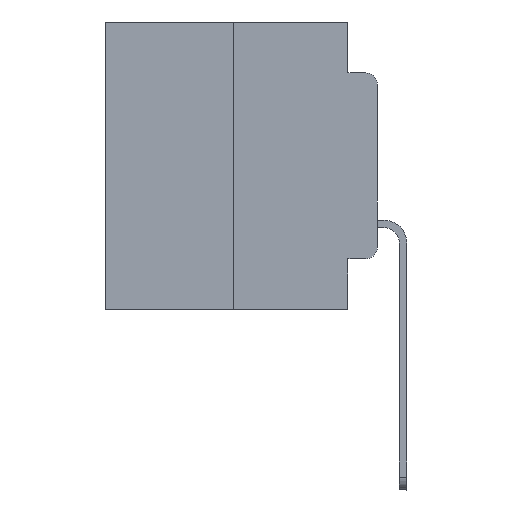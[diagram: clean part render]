
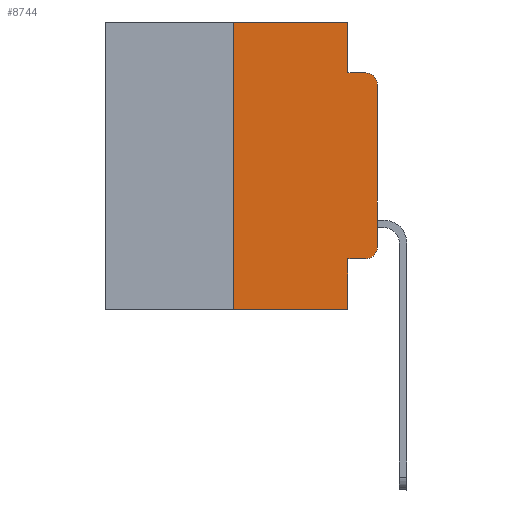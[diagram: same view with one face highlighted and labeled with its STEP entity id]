
A CAD part, left-side view. The second image highlights one B-rep face of the part: STEP entity #8744.
In plain terms, the highlighted planar face has unit normal (-1, 0, 0).
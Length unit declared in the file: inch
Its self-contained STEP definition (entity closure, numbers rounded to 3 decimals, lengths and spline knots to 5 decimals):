
#318 = CARTESIAN_POINT ( 'NONE',  ( 0., 0., -0.3915 ) ) ;
#436 = VERTEX_POINT ( 'NONE', #5753 ) ;
#473 = DIRECTION ( 'NONE',  ( 0., -1., 0. ) ) ;
#689 = CARTESIAN_POINT ( 'NONE',  ( 0., 0.25, 0. ) ) ;
#764 = CARTESIAN_POINT ( 'NONE',  ( 0., 0.02, -0.1085 ) ) ;
#1210 = LINE ( 'NONE', #17907, #14402 ) ;
#1665 = VERTEX_POINT ( 'NONE', #689 ) ;
#1760 = LINE ( 'NONE', #5910, #18018 ) ;
#1878 = EDGE_CURVE ( 'NONE', #26031, #436, #1210, .T. ) ;
#1961 = DIRECTION ( 'NONE',  ( 0., 0., 1. ) ) ;
#2222 = CARTESIAN_POINT ( 'NONE',  ( 0., 0.25, 0. ) ) ;
#2993 = CARTESIAN_POINT ( 'NONE',  ( 0., 0.051, -0.0885 ) ) ;
#3423 = EDGE_CURVE ( 'NONE', #1665, #8297, #6465, .T. ) ;
#4359 = LINE ( 'NONE', #2222, #10262 ) ;
#4571 = DIRECTION ( 'NONE',  ( -1., 0., 0. ) ) ;
#4594 = DIRECTION ( 'NONE',  ( 0., -1., 0. ) ) ;
#4693 = CARTESIAN_POINT ( 'NONE',  ( 0., 0.02, -0.3915 ) ) ;
#5750 = CIRCLE ( 'NONE', #20799, 0.02 ) ;
#5753 = CARTESIAN_POINT ( 'NONE',  ( 0., 0.051, -0.5 ) ) ;
#5910 = CARTESIAN_POINT ( 'NONE',  ( 0., 0., 0. ) ) ;
#6127 = ORIENTED_EDGE ( 'NONE', *, *, #13904, .T. ) ;
#6251 = ORIENTED_EDGE ( 'NONE', *, *, #13626, .T. ) ;
#6265 = ORIENTED_EDGE ( 'NONE', *, *, #24541, .T. ) ;
#6440 = AXIS2_PLACEMENT_3D ( 'NONE', #17855, #13821, #22027 ) ;
#6465 = LINE ( 'NONE', #10780, #17109 ) ;
#6643 = LINE ( 'NONE', #20794, #17611 ) ;
#6711 = CARTESIAN_POINT ( 'NONE',  ( 0., 0.051, -0.0885 ) ) ;
#6777 = VERTEX_POINT ( 'NONE', #6711 ) ;
#7547 = CARTESIAN_POINT ( 'NONE',  ( 0., 0.25, -0.5 ) ) ;
#7629 = EDGE_CURVE ( 'NONE', #23196, #436, #6643, .T. ) ;
#8297 = VERTEX_POINT ( 'NONE', #24075 ) ;
#8603 = AXIS2_PLACEMENT_3D ( 'NONE', #764, #19595, #8967 ) ;
#8744 = ADVANCED_FACE ( 'NONE', ( #24323 ), #26048, .F. ) ;
#8967 = DIRECTION ( 'NONE',  ( 0., 0., -1. ) ) ;
#9240 = CARTESIAN_POINT ( 'NONE',  ( 0., 0.02, -0.4115 ) ) ;
#9968 = DIRECTION ( 'NONE',  ( 0., 0., 1. ) ) ;
#10254 = VERTEX_POINT ( 'NONE', #22483 ) ;
#10262 = VECTOR ( 'NONE', #1961, 39.37008 ) ;
#10688 = LINE ( 'NONE', #18892, #25391 ) ;
#10757 = CIRCLE ( 'NONE', #8603, 0.02 ) ;
#10780 = CARTESIAN_POINT ( 'NONE',  ( 0., 0.473, 0. ) ) ;
#11066 = LINE ( 'NONE', #2993, #14356 ) ;
#11367 = DIRECTION ( 'NONE',  ( 0., 0., -1. ) ) ;
#11372 = EDGE_CURVE ( 'NONE', #8297, #6777, #21191, .T. ) ;
#12203 = VERTEX_POINT ( 'NONE', #9240 ) ;
#12567 = DIRECTION ( 'NONE',  ( 0., -1., 0. ) ) ;
#12688 = ORIENTED_EDGE ( 'NONE', *, *, #24256, .F. ) ;
#12974 = ORIENTED_EDGE ( 'NONE', *, *, #7629, .F. ) ;
#13626 = EDGE_CURVE ( 'NONE', #10254, #17565, #10757, .T. ) ;
#13821 = DIRECTION ( 'NONE',  ( 1., 0., 0. ) ) ;
#13904 = EDGE_CURVE ( 'NONE', #23196, #12203, #10688, .T. ) ;
#14356 = VECTOR ( 'NONE', #4594, 39.37008 ) ;
#14402 = VECTOR ( 'NONE', #23706, 39.37008 ) ;
#16781 = EDGE_CURVE ( 'NONE', #6777, #17565, #11066, .T. ) ;
#17099 = DIRECTION ( 'NONE',  ( 0., 0., -1. ) ) ;
#17109 = VECTOR ( 'NONE', #12567, 39.37008 ) ;
#17238 = EDGE_CURVE ( 'NONE', #12203, #22570, #5750, .T. ) ;
#17565 = VERTEX_POINT ( 'NONE', #18771 ) ;
#17611 = VECTOR ( 'NONE', #24832, 39.37008 ) ;
#17855 = CARTESIAN_POINT ( 'NONE',  ( 0., 0.473, 0. ) ) ;
#17907 = CARTESIAN_POINT ( 'NONE',  ( 0., 0.473, -0.5 ) ) ;
#18018 = VECTOR ( 'NONE', #9968, 39.37008 ) ;
#18771 = CARTESIAN_POINT ( 'NONE',  ( 0., 0.02, -0.0885 ) ) ;
#18892 = CARTESIAN_POINT ( 'NONE',  ( 0., 0.051, -0.4115 ) ) ;
#19398 = VECTOR ( 'NONE', #11367, 39.37008 ) ;
#19595 = DIRECTION ( 'NONE',  ( -1., 0., 0. ) ) ;
#20135 = ORIENTED_EDGE ( 'NONE', *, *, #3423, .F. ) ;
#20196 = EDGE_LOOP ( 'NONE', ( #6265, #6251, #22296, #20883, #20135, #12688, #24653, #12974, #6127, #25940 ) ) ;
#20794 = CARTESIAN_POINT ( 'NONE',  ( 0., 0.051, 0. ) ) ;
#20799 = AXIS2_PLACEMENT_3D ( 'NONE', #4693, #4571, #17099 ) ;
#20883 = ORIENTED_EDGE ( 'NONE', *, *, #11372, .F. ) ;
#21191 = LINE ( 'NONE', #25227, #19398 ) ;
#22027 = DIRECTION ( 'NONE',  ( 0., 0., -1. ) ) ;
#22296 = ORIENTED_EDGE ( 'NONE', *, *, #16781, .F. ) ;
#22483 = CARTESIAN_POINT ( 'NONE',  ( 0., 0., -0.1085 ) ) ;
#22570 = VERTEX_POINT ( 'NONE', #318 ) ;
#23196 = VERTEX_POINT ( 'NONE', #23568 ) ;
#23568 = CARTESIAN_POINT ( 'NONE',  ( 0., 0.051, -0.4115 ) ) ;
#23706 = DIRECTION ( 'NONE',  ( 0., -1., 0. ) ) ;
#24075 = CARTESIAN_POINT ( 'NONE',  ( 0., 0.051, 0. ) ) ;
#24256 = EDGE_CURVE ( 'NONE', #26031, #1665, #4359, .T. ) ;
#24323 = FACE_OUTER_BOUND ( 'NONE', #20196, .T. ) ;
#24541 = EDGE_CURVE ( 'NONE', #22570, #10254, #1760, .T. ) ;
#24653 = ORIENTED_EDGE ( 'NONE', *, *, #1878, .T. ) ;
#24832 = DIRECTION ( 'NONE',  ( 0., 0., -1. ) ) ;
#25227 = CARTESIAN_POINT ( 'NONE',  ( 0., 0.051, 0. ) ) ;
#25391 = VECTOR ( 'NONE', #473, 39.37008 ) ;
#25940 = ORIENTED_EDGE ( 'NONE', *, *, #17238, .T. ) ;
#26031 = VERTEX_POINT ( 'NONE', #7547 ) ;
#26048 = PLANE ( 'NONE',  #6440 ) ;
